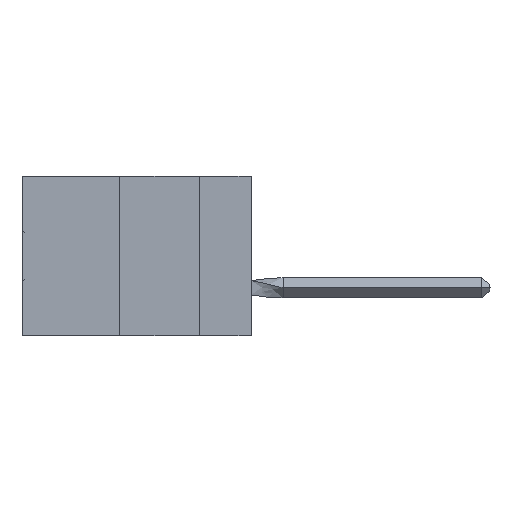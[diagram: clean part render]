
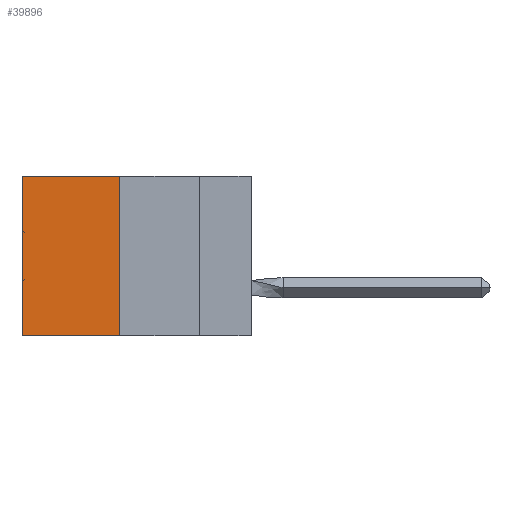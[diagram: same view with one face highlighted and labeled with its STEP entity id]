
A CAD part, left-side view. The second image highlights one B-rep face of the part: STEP entity #39896.
In plain terms, the highlighted planar face has unit normal (-1, 0, 0).
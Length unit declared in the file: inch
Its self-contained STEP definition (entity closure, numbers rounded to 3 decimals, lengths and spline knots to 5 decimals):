
#209 = VECTOR ( 'NONE', #15095, 39.37008 ) ;
#4323 = DIRECTION ( 'NONE',  ( 0., 1., 0. ) ) ;
#8825 = CARTESIAN_POINT ( 'NONE',  ( 0.305, 0.413, 0. ) ) ;
#9976 = EDGE_CURVE ( 'NONE', #42699, #32616, #40053, .T. ) ;
#10233 = CARTESIAN_POINT ( 'NONE',  ( 0.305, 0.72, -0.5 ) ) ;
#11813 = LINE ( 'NONE', #39300, #31300 ) ;
#13750 = PLANE ( 'NONE',  #21241 ) ;
#13976 = CARTESIAN_POINT ( 'NONE',  ( 0.305, 0.72, -0.5 ) ) ;
#14581 = CARTESIAN_POINT ( 'NONE',  ( 0.305, 0.413, -0.5 ) ) ;
#15095 = DIRECTION ( 'NONE',  ( 0., 0., -1. ) ) ;
#17102 = ORIENTED_EDGE ( 'NONE', *, *, #9976, .T. ) ;
#17502 = EDGE_LOOP ( 'NONE', ( #17102, #22778, #20641, #31701 ) ) ;
#18556 = EDGE_CURVE ( 'NONE', #33037, #34806, #42933, .T. ) ;
#18676 = CARTESIAN_POINT ( 'NONE',  ( 0.305, 0.413, -0.5 ) ) ;
#19784 = DIRECTION ( 'NONE',  ( 0., 1., 0. ) ) ;
#20641 = ORIENTED_EDGE ( 'NONE', *, *, #18556, .F. ) ;
#21241 = AXIS2_PLACEMENT_3D ( 'NONE', #25187, #36794, #40519 ) ;
#22778 = ORIENTED_EDGE ( 'NONE', *, *, #40227, .F. ) ;
#25162 = LINE ( 'NONE', #47352, #38573 ) ;
#25187 = CARTESIAN_POINT ( 'NONE',  ( 0.305, 0.413, -0.5 ) ) ;
#25725 = CARTESIAN_POINT ( 'NONE',  ( 0.305, 0.72, 0. ) ) ;
#26701 = EDGE_CURVE ( 'NONE', #33037, #42699, #25162, .T. ) ;
#31300 = VECTOR ( 'NONE', #4323, 39.37008 ) ;
#31701 = ORIENTED_EDGE ( 'NONE', *, *, #26701, .T. ) ;
#32616 = VERTEX_POINT ( 'NONE', #13976 ) ;
#33037 = VERTEX_POINT ( 'NONE', #8825 ) ;
#34806 = VERTEX_POINT ( 'NONE', #14581 ) ;
#36794 = DIRECTION ( 'NONE',  ( 1., 0., 0. ) ) ;
#38573 = VECTOR ( 'NONE', #19784, 39.37008 ) ;
#39300 = CARTESIAN_POINT ( 'NONE',  ( 0.305, 0.413, -0.5 ) ) ;
#39896 = ADVANCED_FACE ( 'NONE', ( #41769 ), #13750, .F. ) ;
#40053 = LINE ( 'NONE', #10233, #49214 ) ;
#40227 = EDGE_CURVE ( 'NONE', #34806, #32616, #11813, .T. ) ;
#40519 = DIRECTION ( 'NONE',  ( 0., 0., -1. ) ) ;
#41769 = FACE_OUTER_BOUND ( 'NONE', #17502, .T. ) ;
#41782 = DIRECTION ( 'NONE',  ( 0., 0., -1. ) ) ;
#42699 = VERTEX_POINT ( 'NONE', #25725 ) ;
#42933 = LINE ( 'NONE', #18676, #209 ) ;
#47352 = CARTESIAN_POINT ( 'NONE',  ( 0.305, 0.413, 0. ) ) ;
#49214 = VECTOR ( 'NONE', #41782, 39.37008 ) ;
